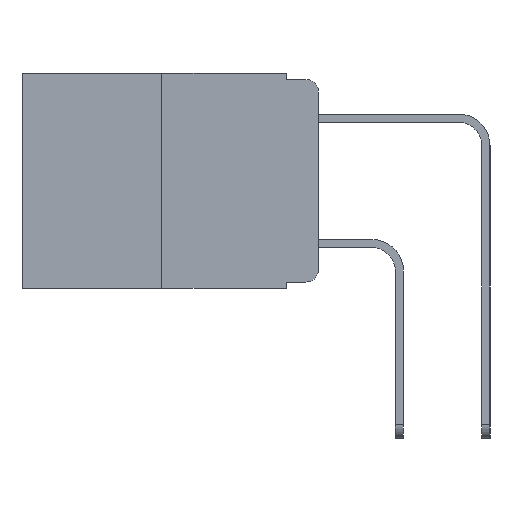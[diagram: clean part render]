
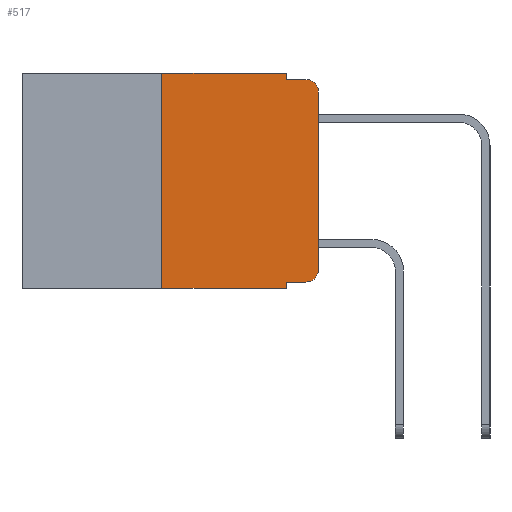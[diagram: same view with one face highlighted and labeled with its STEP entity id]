
A CAD part, left-side view. The second image highlights one B-rep face of the part: STEP entity #517.
In plain terms, the highlighted planar face has unit normal (-1, 0, 0).
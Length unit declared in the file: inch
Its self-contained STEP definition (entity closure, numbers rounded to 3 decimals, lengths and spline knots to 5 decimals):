
#216 = VERTEX_POINT ( 'NONE', #8245 ) ;
#225 = VERTEX_POINT ( 'NONE', #8511 ) ;
#357 = AXIS2_PLACEMENT_3D ( 'NONE', #14416, #12905, #12820 ) ;
#517 = ADVANCED_FACE ( 'NONE', ( #9658 ), #12925, .F. ) ;
#1067 = VECTOR ( 'NONE', #6805, 39.37008 ) ;
#1370 = CARTESIAN_POINT ( 'NONE',  ( 0., 0., 0. ) ) ;
#1449 = EDGE_CURVE ( 'NONE', #7958, #11099, #5814, .T. ) ;
#1571 = CARTESIAN_POINT ( 'NONE',  ( 0., 0.051, 0. ) ) ;
#1752 = VECTOR ( 'NONE', #11581, 39.37008 ) ;
#1773 = VECTOR ( 'NONE', #2998, 39.37008 ) ;
#2009 = DIRECTION ( 'NONE',  ( -1., 0., 0. ) ) ;
#2035 = VECTOR ( 'NONE', #12142, 39.37008 ) ;
#2730 = EDGE_CURVE ( 'NONE', #4337, #225, #14451, .T. ) ;
#2869 = ORIENTED_EDGE ( 'NONE', *, *, #6979, .F. ) ;
#2998 = DIRECTION ( 'NONE',  ( 0., 0., -1. ) ) ;
#3418 = CARTESIAN_POINT ( 'NONE',  ( 0., 0.473, -0.343 ) ) ;
#3794 = EDGE_CURVE ( 'NONE', #6789, #216, #8547, .T. ) ;
#4275 = LINE ( 'NONE', #12228, #1067 ) ;
#4337 = VERTEX_POINT ( 'NONE', #13092 ) ;
#4357 = CARTESIAN_POINT ( 'NONE',  ( 0., 0.473, 0. ) ) ;
#4548 = AXIS2_PLACEMENT_3D ( 'NONE', #8912, #2009, #10004 ) ;
#4613 = DIRECTION ( 'NONE',  ( 0., -1., 0. ) ) ;
#4679 = DIRECTION ( 'NONE',  ( 0., -1., 0. ) ) ;
#5146 = DIRECTION ( 'NONE',  ( 0., 0., -1. ) ) ;
#5156 = LINE ( 'NONE', #3418, #11074 ) ;
#5279 = ORIENTED_EDGE ( 'NONE', *, *, #13952, .F. ) ;
#5602 = CIRCLE ( 'NONE', #6684, 0.02 ) ;
#5638 = ORIENTED_EDGE ( 'NONE', *, *, #3794, .F. ) ;
#5814 = LINE ( 'NONE', #1571, #11358 ) ;
#5892 = CARTESIAN_POINT ( 'NONE',  ( 0., 0.25, -0.343 ) ) ;
#6074 = CARTESIAN_POINT ( 'NONE',  ( 0., 0.051, -0.01 ) ) ;
#6684 = AXIS2_PLACEMENT_3D ( 'NONE', #12302, #11776, #5146 ) ;
#6721 = ORIENTED_EDGE ( 'NONE', *, *, #1449, .F. ) ;
#6789 = VERTEX_POINT ( 'NONE', #7695 ) ;
#6805 = DIRECTION ( 'NONE',  ( 0., 0., 1. ) ) ;
#6979 = EDGE_CURVE ( 'NONE', #8689, #6789, #4275, .T. ) ;
#7247 = ORIENTED_EDGE ( 'NONE', *, *, #11312, .T. ) ;
#7695 = CARTESIAN_POINT ( 'NONE',  ( 0., 0.25, 0. ) ) ;
#7728 = EDGE_CURVE ( 'NONE', #8689, #11099, #5156, .T. ) ;
#7924 = LINE ( 'NONE', #10245, #12992 ) ;
#7958 = VERTEX_POINT ( 'NONE', #13672 ) ;
#8245 = CARTESIAN_POINT ( 'NONE',  ( 0., 0.051, 0. ) ) ;
#8276 = ORIENTED_EDGE ( 'NONE', *, *, #9183, .F. ) ;
#8278 = LINE ( 'NONE', #6074, #1752 ) ;
#8332 = DIRECTION ( 'NONE',  ( 0., 0., 1. ) ) ;
#8463 = EDGE_LOOP ( 'NONE', ( #12658, #7247, #5279, #8276, #5638, #2869, #9304, #6721, #9662, #9992 ) ) ;
#8470 = LINE ( 'NONE', #1370, #13855 ) ;
#8511 = CARTESIAN_POINT ( 'NONE',  ( 0., 0., -0.313 ) ) ;
#8547 = LINE ( 'NONE', #4357, #2035 ) ;
#8689 = VERTEX_POINT ( 'NONE', #5892 ) ;
#8831 = EDGE_CURVE ( 'NONE', #225, #10972, #8470, .T. ) ;
#8912 = CARTESIAN_POINT ( 'NONE',  ( 0., 0.02, -0.313 ) ) ;
#9183 = EDGE_CURVE ( 'NONE', #216, #10231, #13683, .T. ) ;
#9304 = ORIENTED_EDGE ( 'NONE', *, *, #7728, .T. ) ;
#9475 = CARTESIAN_POINT ( 'NONE',  ( 0., 0.02, -0.01 ) ) ;
#9658 = FACE_OUTER_BOUND ( 'NONE', #8463, .T. ) ;
#9662 = ORIENTED_EDGE ( 'NONE', *, *, #14476, .T. ) ;
#9818 = CARTESIAN_POINT ( 'NONE',  ( 0., 0.051, 0. ) ) ;
#9992 = ORIENTED_EDGE ( 'NONE', *, *, #2730, .T. ) ;
#10004 = DIRECTION ( 'NONE',  ( 0., 0., -1. ) ) ;
#10015 = CARTESIAN_POINT ( 'NONE',  ( 0., 0., -0.03 ) ) ;
#10231 = VERTEX_POINT ( 'NONE', #14415 ) ;
#10245 = CARTESIAN_POINT ( 'NONE',  ( 0., 0.051, -0.333 ) ) ;
#10972 = VERTEX_POINT ( 'NONE', #10015 ) ;
#11074 = VECTOR ( 'NONE', #4613, 39.37008 ) ;
#11099 = VERTEX_POINT ( 'NONE', #13610 ) ;
#11312 = EDGE_CURVE ( 'NONE', #10972, #14017, #5602, .T. ) ;
#11358 = VECTOR ( 'NONE', #13355, 39.37008 ) ;
#11581 = DIRECTION ( 'NONE',  ( 0., -1., 0. ) ) ;
#11776 = DIRECTION ( 'NONE',  ( -1., 0., 0. ) ) ;
#12142 = DIRECTION ( 'NONE',  ( 0., -1., 0. ) ) ;
#12228 = CARTESIAN_POINT ( 'NONE',  ( 0., 0.25, 0. ) ) ;
#12302 = CARTESIAN_POINT ( 'NONE',  ( 0., 0.02, -0.03 ) ) ;
#12658 = ORIENTED_EDGE ( 'NONE', *, *, #8831, .T. ) ;
#12820 = DIRECTION ( 'NONE',  ( 0., 0., -1. ) ) ;
#12905 = DIRECTION ( 'NONE',  ( 1., 0., 0. ) ) ;
#12925 = PLANE ( 'NONE',  #357 ) ;
#12992 = VECTOR ( 'NONE', #4679, 39.37008 ) ;
#13092 = CARTESIAN_POINT ( 'NONE',  ( 0., 0.02, -0.333 ) ) ;
#13355 = DIRECTION ( 'NONE',  ( 0., 0., -1. ) ) ;
#13610 = CARTESIAN_POINT ( 'NONE',  ( 0., 0.051, -0.343 ) ) ;
#13672 = CARTESIAN_POINT ( 'NONE',  ( 0., 0.051, -0.333 ) ) ;
#13683 = LINE ( 'NONE', #9818, #1773 ) ;
#13855 = VECTOR ( 'NONE', #8332, 39.37008 ) ;
#13952 = EDGE_CURVE ( 'NONE', #10231, #14017, #8278, .T. ) ;
#14017 = VERTEX_POINT ( 'NONE', #9475 ) ;
#14415 = CARTESIAN_POINT ( 'NONE',  ( 0., 0.051, -0.01 ) ) ;
#14416 = CARTESIAN_POINT ( 'NONE',  ( 0., 0.473, 0. ) ) ;
#14451 = CIRCLE ( 'NONE', #4548, 0.02 ) ;
#14476 = EDGE_CURVE ( 'NONE', #7958, #4337, #7924, .T. ) ;
